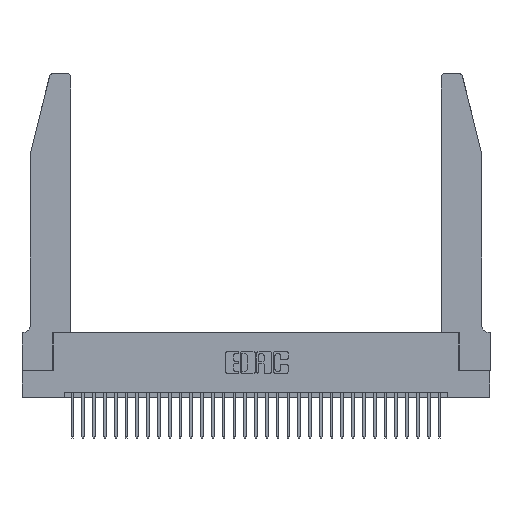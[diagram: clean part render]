
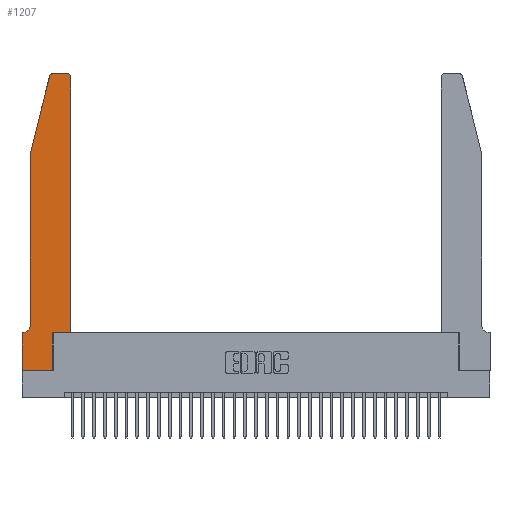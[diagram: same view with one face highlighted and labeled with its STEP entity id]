
A CAD part, top view. The second image highlights one B-rep face of the part: STEP entity #1207.
In plain terms, the highlighted planar face has unit normal (0, 0, 1).
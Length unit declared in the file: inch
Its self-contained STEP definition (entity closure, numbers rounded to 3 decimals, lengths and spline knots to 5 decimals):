
#288 = ORIENTED_EDGE ( 'NONE', *, *, #22224, .T. ) ;
#718 = ORIENTED_EDGE ( 'NONE', *, *, #16617, .T. ) ;
#1207 = ADVANCED_FACE ( 'NONE', ( #9285 ), #32201, .T. ) ;
#2032 = DIRECTION ( 'NONE',  ( 0., 0., 1. ) ) ;
#2088 = AXIS2_PLACEMENT_3D ( 'NONE', #26273, #20786, #13001 ) ;
#2353 = DIRECTION ( 'NONE',  ( 1., 0., 0. ) ) ;
#2605 = VERTEX_POINT ( 'NONE', #28354 ) ;
#2756 = VERTEX_POINT ( 'NONE', #15395 ) ;
#2923 = CARTESIAN_POINT ( 'NONE',  ( 0.4205, 2.72, 0.37 ) ) ;
#3198 = DIRECTION ( 'NONE',  ( 0., -1., 0. ) ) ;
#3430 = EDGE_CURVE ( 'NONE', #31028, #2756, #30818, .T. ) ;
#3731 = EDGE_CURVE ( 'NONE', #23547, #20437, #6301, .T. ) ;
#5577 = VERTEX_POINT ( 'NONE', #8865 ) ;
#5898 = CARTESIAN_POINT ( 'NONE',  ( 0., 0.35, 0.37 ) ) ;
#6255 = VECTOR ( 'NONE', #16587, 39.37008 ) ;
#6301 = LINE ( 'NONE', #17240, #28448 ) ;
#6352 = CARTESIAN_POINT ( 'NONE',  ( 0.2865, 0.35, 0.37 ) ) ;
#6624 = DIRECTION ( 'NONE',  ( 1., 0., 0. ) ) ;
#6870 = ORIENTED_EDGE ( 'NONE', *, *, #8169, .T. ) ;
#7247 = EDGE_CURVE ( 'NONE', #19332, #9936, #24850, .T. ) ;
#7255 = DIRECTION ( 'NONE',  ( 0., 1., 0. ) ) ;
#7526 = CARTESIAN_POINT ( 'NONE',  ( 0.4505, 2.72, 0.37 ) ) ;
#7965 = ORIENTED_EDGE ( 'NONE', *, *, #18744, .T. ) ;
#8169 = EDGE_CURVE ( 'NONE', #14932, #2605, #18310, .T. ) ;
#8263 = ORIENTED_EDGE ( 'NONE', *, *, #11045, .T. ) ;
#8865 = CARTESIAN_POINT ( 'NONE',  ( 0.284, 2.75, 0.37 ) ) ;
#9285 = FACE_OUTER_BOUND ( 'NONE', #27053, .T. ) ;
#9694 = LINE ( 'NONE', #28234, #16127 ) ;
#9832 = CARTESIAN_POINT ( 'NONE',  ( 0.4505, 0.35, 0.37 ) ) ;
#9900 = LINE ( 'NONE', #6352, #6255 ) ;
#9936 = VERTEX_POINT ( 'NONE', #19867 ) ;
#9955 = CARTESIAN_POINT ( 'NONE',  ( 0.0755, 0.35, 0.37 ) ) ;
#9967 = CARTESIAN_POINT ( 'NONE',  ( 0.2865, 0., 0.37 ) ) ;
#9972 = CARTESIAN_POINT ( 'NONE',  ( 0.0755, 2., 0.37 ) ) ;
#11045 = EDGE_CURVE ( 'NONE', #5577, #14932, #19811, .T. ) ;
#11107 = CARTESIAN_POINT ( 'NONE',  ( 0.4505, 0.35, 0.37 ) ) ;
#11288 = CARTESIAN_POINT ( 'NONE',  ( 0.0755, 2., 0.37 ) ) ;
#11391 = VECTOR ( 'NONE', #7255, 39.37008 ) ;
#11705 = VECTOR ( 'NONE', #12423, 39.37008 ) ;
#12075 = CARTESIAN_POINT ( 'NONE',  ( 0.0055, 0.35, 0.37 ) ) ;
#12238 = CARTESIAN_POINT ( 'NONE',  ( 0.2605, 2.75, 0.37 ) ) ;
#12423 = DIRECTION ( 'NONE',  ( -1., 0., 0. ) ) ;
#12699 = CARTESIAN_POINT ( 'NONE',  ( 0.0755, 0.42, 0.37 ) ) ;
#12704 = ORIENTED_EDGE ( 'NONE', *, *, #16071, .T. ) ;
#13001 = DIRECTION ( 'NONE',  ( -1., 0., 0. ) ) ;
#13271 = EDGE_CURVE ( 'NONE', #14785, #21227, #18784, .T. ) ;
#13719 = CARTESIAN_POINT ( 'NONE',  ( 0.2865, 0.35, 0.37 ) ) ;
#14044 = ORIENTED_EDGE ( 'NONE', *, *, #3430, .T. ) ;
#14179 = DIRECTION ( 'NONE',  ( 0., 0., 1. ) ) ;
#14562 = LINE ( 'NONE', #12238, #30210 ) ;
#14669 = CARTESIAN_POINT ( 'NONE',  ( 0.25487, 2.72718, 0.37 ) ) ;
#14671 = DIRECTION ( 'NONE',  ( 0., -1., 0. ) ) ;
#14785 = VERTEX_POINT ( 'NONE', #12699 ) ;
#14932 = VERTEX_POINT ( 'NONE', #14669 ) ;
#15395 = CARTESIAN_POINT ( 'NONE',  ( 0.4505, 0.35, 0.37 ) ) ;
#15697 = ORIENTED_EDGE ( 'NONE', *, *, #31899, .T. ) ;
#16015 = LINE ( 'NONE', #11288, #21696 ) ;
#16071 = EDGE_CURVE ( 'NONE', #9936, #5577, #14562, .T. ) ;
#16127 = VECTOR ( 'NONE', #23083, 39.37008 ) ;
#16133 = ORIENTED_EDGE ( 'NONE', *, *, #23652, .T. ) ;
#16587 = DIRECTION ( 'NONE',  ( 0., 1., 0. ) ) ;
#16617 = EDGE_CURVE ( 'NONE', #20437, #20672, #9694, .T. ) ;
#16970 = CARTESIAN_POINT ( 'NONE',  ( 0., 0.35, 0.37 ) ) ;
#17180 = VECTOR ( 'NONE', #18875, 39.37008 ) ;
#17240 = CARTESIAN_POINT ( 'NONE',  ( 0., 0., 0.37 ) ) ;
#17389 = DIRECTION ( 'NONE',  ( -1., 0., 0. ) ) ;
#17405 = LINE ( 'NONE', #9832, #11391 ) ;
#18310 = LINE ( 'NONE', #9972, #33144 ) ;
#18744 = EDGE_CURVE ( 'NONE', #2756, #19332, #17405, .T. ) ;
#18784 = CIRCLE ( 'NONE', #2088, 0.07 ) ;
#18875 = DIRECTION ( 'NONE',  ( 1., 0., 0. ) ) ;
#19332 = VERTEX_POINT ( 'NONE', #7526 ) ;
#19811 = CIRCLE ( 'NONE', #27893, 0.03 ) ;
#19867 = CARTESIAN_POINT ( 'NONE',  ( 0.4205, 2.75, 0.37 ) ) ;
#20437 = VERTEX_POINT ( 'NONE', #31295 ) ;
#20563 = LINE ( 'NONE', #9955, #11705 ) ;
#20672 = VERTEX_POINT ( 'NONE', #9967 ) ;
#20786 = DIRECTION ( 'NONE',  ( 0., 0., -1. ) ) ;
#21043 = DIRECTION ( 'NONE',  ( 1., 0., 0. ) ) ;
#21227 = VERTEX_POINT ( 'NONE', #12075 ) ;
#21696 = VECTOR ( 'NONE', #3198, 39.37008 ) ;
#22224 = EDGE_CURVE ( 'NONE', #2605, #14785, #16015, .T. ) ;
#23083 = DIRECTION ( 'NONE',  ( 1., 0., 0. ) ) ;
#23547 = VERTEX_POINT ( 'NONE', #5898 ) ;
#23652 = EDGE_CURVE ( 'NONE', #20672, #31028, #9900, .T. ) ;
#24607 = AXIS2_PLACEMENT_3D ( 'NONE', #2923, #28664, #21043 ) ;
#24850 = CIRCLE ( 'NONE', #24607, 0.03 ) ;
#24976 = ORIENTED_EDGE ( 'NONE', *, *, #13271, .T. ) ;
#25493 = DIRECTION ( 'NONE',  ( -0.239, -0.971, 0. ) ) ;
#26273 = CARTESIAN_POINT ( 'NONE',  ( 0.0055, 0.42, 0.37 ) ) ;
#27053 = EDGE_LOOP ( 'NONE', ( #12704, #8263, #6870, #288, #24976, #15697, #28233, #718, #16133, #14044, #7965, #27097 ) ) ;
#27097 = ORIENTED_EDGE ( 'NONE', *, *, #7247, .T. ) ;
#27893 = AXIS2_PLACEMENT_3D ( 'NONE', #30319, #2032, #2353 ) ;
#28233 = ORIENTED_EDGE ( 'NONE', *, *, #3731, .T. ) ;
#28234 = CARTESIAN_POINT ( 'NONE',  ( 0., 0., 0.37 ) ) ;
#28354 = CARTESIAN_POINT ( 'NONE',  ( 0.0755, 2., 0.37 ) ) ;
#28448 = VECTOR ( 'NONE', #14671, 39.37008 ) ;
#28664 = DIRECTION ( 'NONE',  ( 0., 0., 1. ) ) ;
#30210 = VECTOR ( 'NONE', #17389, 39.37008 ) ;
#30319 = CARTESIAN_POINT ( 'NONE',  ( 0.284, 2.72, 0.37 ) ) ;
#30818 = LINE ( 'NONE', #11107, #17180 ) ;
#31028 = VERTEX_POINT ( 'NONE', #13719 ) ;
#31295 = CARTESIAN_POINT ( 'NONE',  ( 0., 0., 0.37 ) ) ;
#31331 = AXIS2_PLACEMENT_3D ( 'NONE', #16970, #14179, #6624 ) ;
#31899 = EDGE_CURVE ( 'NONE', #21227, #23547, #20563, .T. ) ;
#32201 = PLANE ( 'NONE',  #31331 ) ;
#33144 = VECTOR ( 'NONE', #25493, 39.37008 ) ;
